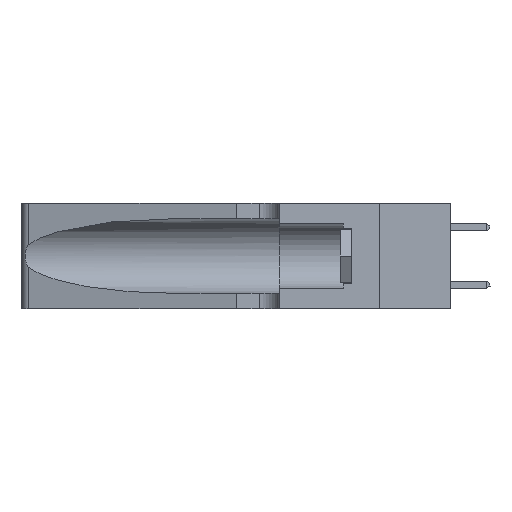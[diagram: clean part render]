
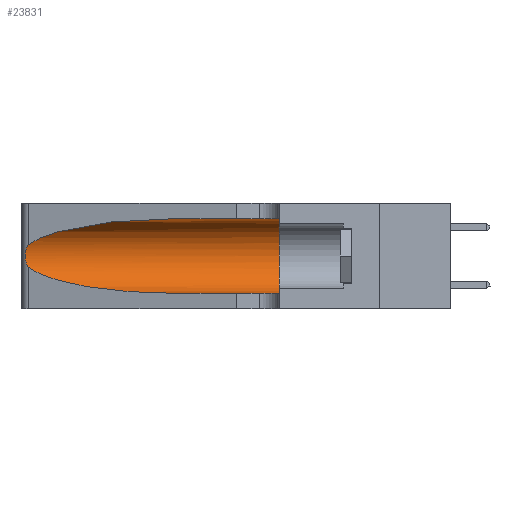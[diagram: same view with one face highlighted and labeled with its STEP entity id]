
A CAD part, left-side view. The second image highlights one B-rep face of the part: STEP entity #23831.
In plain terms, the highlighted cylindrical face has radius 3.308 mm (diameter 6.617 mm), a partial arc.
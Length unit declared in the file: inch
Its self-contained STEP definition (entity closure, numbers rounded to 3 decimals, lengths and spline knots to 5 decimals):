
#140 = ORIENTED_EDGE ( 'NONE', *, *, #17672, .T. ) ;
#595 = B_SPLINE_CURVE_WITH_KNOTS ( 'NONE', 3,
 ( #10489, #21453, #28916, #2575, #16901, #21864, #9823, #29399, #17494, #22380, #30138, #13335, #4917, #28024 ),
 .UNSPECIFIED., .F., .F.,
 ( 4, 2, 2, 2, 2, 2, 4 ),
 ( 0., 0.00027, 0.00053, 0.00107, 0.0016, 0.00187, 0.00214 ),
 .UNSPECIFIED. ) ;
#686 = AXIS2_PLACEMENT_3D ( 'NONE', #2015, #11781, #25969 ) ;
#1318 = DIRECTION ( 'NONE',  ( 0., -1., 0. ) ) ;
#2015 = CARTESIAN_POINT ( 'NONE',  ( 0.1305, 1.61858, 0.185 ) ) ;
#2575 = CARTESIAN_POINT ( 'NONE',  ( 0.25787, 1.23484, 0.2124 ) ) ;
#3003 = EDGE_CURVE ( 'NONE', #3062, #8077, #16584, .T. ) ;
#3062 = VERTEX_POINT ( 'NONE', #16203 ) ;
#3171 = ORIENTED_EDGE ( 'NONE', *, *, #3003, .F. ) ;
#3397 = VERTEX_POINT ( 'NONE', #16098 ) ;
#4917 = CARTESIAN_POINT ( 'NONE',  ( 0.25555, 1.22993, 0.14849 ) ) ;
#7480 = AXIS2_PLACEMENT_3D ( 'NONE', #28625, #30835, #21142 ) ;
#7861 = DIRECTION ( 'NONE',  ( 0., -1., 0. ) ) ;
#8012 = CARTESIAN_POINT ( 'NONE',  ( 0.2373, 1.15595, 0.28018 ) ) ;
#8077 = VERTEX_POINT ( 'NONE', #28107 ) ;
#8131 = CARTESIAN_POINT ( 'NONE',  ( 0.25487, 1.22718, 0.22369 ) ) ;
#8479 = CARTESIAN_POINT ( 'NONE',  ( 0.1305, 1.61858, 0.31525 ) ) ;
#9499 =( BOUNDED_CURVE ( )  B_SPLINE_CURVE ( 3, ( #11770, #10043, #17106, #12783 ),
 .UNSPECIFIED., .F., .T. ) 
 B_SPLINE_CURVE_WITH_KNOTS ( ( 4, 4 ),
 ( 3.44316, 4.71239 ),
 .UNSPECIFIED. ) 
 CURVE ( )  GEOMETRIC_REPRESENTATION_ITEM ( )  RATIONAL_B_SPLINE_CURVE ( ( 1., 0.87, 0.87, 1. ) ) 
 REPRESENTATION_ITEM ( '' )  );
#9823 = CARTESIAN_POINT ( 'NONE',  ( 0.26075, 1.23896, 0.19203 ) ) ;
#10043 = CARTESIAN_POINT ( 'NONE',  ( 0.2373, 1.15595, 0.08982 ) ) ;
#10489 = CARTESIAN_POINT ( 'NONE',  ( 0.25487, 1.22718, 0.22369 ) ) ;
#11770 = CARTESIAN_POINT ( 'NONE',  ( 0.25487, 1.22718, 0.14631 ) ) ;
#11781 = DIRECTION ( 'NONE',  ( 0., -1., 0. ) ) ;
#12393 = VECTOR ( 'NONE', #7861, 39.37008 ) ;
#12783 = CARTESIAN_POINT ( 'NONE',  ( 0.1305, 0.72297, 0.05475 ) ) ;
#13335 = CARTESIAN_POINT ( 'NONE',  ( 0.25639, 1.23186, 0.15144 ) ) ;
#13551 = EDGE_CURVE ( 'NONE', #17239, #24078, #9499, .T. ) ;
#13596 = ORIENTED_EDGE ( 'NONE', *, *, #28019, .T. ) ;
#14222 = EDGE_CURVE ( 'NONE', #3397, #3062, #29926, .T. ) ;
#15658 = CARTESIAN_POINT ( 'NONE',  ( 0.1305, 0.72297, 0.05475 ) ) ;
#16098 = CARTESIAN_POINT ( 'NONE',  ( 0.1305, 0.72297, 0.31525 ) ) ;
#16203 = CARTESIAN_POINT ( 'NONE',  ( 0.1305, 0.35, 0.31525 ) ) ;
#16584 = CIRCLE ( 'NONE', #7480, 0.13025 ) ;
#16759 = CYLINDRICAL_SURFACE ( 'NONE', #686, 0.13025 ) ;
#16901 = CARTESIAN_POINT ( 'NONE',  ( 0.25854, 1.2359, 0.20912 ) ) ;
#17106 = CARTESIAN_POINT ( 'NONE',  ( 0.18966, 0.96281, 0.05475 ) ) ;
#17239 = VERTEX_POINT ( 'NONE', #25004 ) ;
#17494 = CARTESIAN_POINT ( 'NONE',  ( 0.26017, 1.23833, 0.17102 ) ) ;
#17672 = EDGE_CURVE ( 'NONE', #20679, #17239, #595, .T. ) ;
#18818 = LINE ( 'NONE', #22119, #12393 ) ;
#20454 = CARTESIAN_POINT ( 'NONE',  ( 0.1305, 0.72297, 0.31525 ) ) ;
#20679 = VERTEX_POINT ( 'NONE', #21234 ) ;
#20859 = EDGE_LOOP ( 'NONE', ( #23360, #140, #28391, #13596, #3171, #23961 ) ) ;
#21142 = DIRECTION ( 'NONE',  ( 0., 0., 1. ) ) ;
#21234 = CARTESIAN_POINT ( 'NONE',  ( 0.25487, 1.22718, 0.22369 ) ) ;
#21453 = CARTESIAN_POINT ( 'NONE',  ( 0.25555, 1.22994, 0.2215 ) ) ;
#21864 = CARTESIAN_POINT ( 'NONE',  ( 0.26018, 1.23835, 0.19895 ) ) ;
#22119 = CARTESIAN_POINT ( 'NONE',  ( 0.1305, 1.61858, 0.05475 ) ) ;
#22380 = CARTESIAN_POINT ( 'NONE',  ( 0.25856, 1.23593, 0.16098 ) ) ;
#22589 = CARTESIAN_POINT ( 'NONE',  ( 0.18966, 0.96281, 0.31525 ) ) ;
#23360 = ORIENTED_EDGE ( 'NONE', *, *, #23929, .T. ) ;
#23831 = ADVANCED_FACE ( 'NONE', ( #29248 ), #16759, .F. ) ;
#23929 = EDGE_CURVE ( 'NONE', #3397, #20679, #25993, .T. ) ;
#23961 = ORIENTED_EDGE ( 'NONE', *, *, #14222, .F. ) ;
#24078 = VERTEX_POINT ( 'NONE', #15658 ) ;
#25004 = CARTESIAN_POINT ( 'NONE',  ( 0.25487, 1.22718, 0.14631 ) ) ;
#25969 = DIRECTION ( 'NONE',  ( 0., 0., -1. ) ) ;
#25993 =( BOUNDED_CURVE ( )  B_SPLINE_CURVE ( 3, ( #20454, #22589, #8012, #8131 ),
 .UNSPECIFIED., .F., .F. ) 
 B_SPLINE_CURVE_WITH_KNOTS ( ( 4, 4 ),
 ( 1.5708, 2.84003 ),
 .UNSPECIFIED. ) 
 CURVE ( )  GEOMETRIC_REPRESENTATION_ITEM ( )  RATIONAL_B_SPLINE_CURVE ( ( 1., 0.87, 0.87, 1. ) ) 
 REPRESENTATION_ITEM ( '' )  );
#26533 = VECTOR ( 'NONE', #1318, 39.37008 ) ;
#28019 = EDGE_CURVE ( 'NONE', #24078, #8077, #18818, .T. ) ;
#28024 = CARTESIAN_POINT ( 'NONE',  ( 0.25487, 1.22718, 0.14631 ) ) ;
#28107 = CARTESIAN_POINT ( 'NONE',  ( 0.1305, 0.35, 0.05475 ) ) ;
#28391 = ORIENTED_EDGE ( 'NONE', *, *, #13551, .T. ) ;
#28625 = CARTESIAN_POINT ( 'NONE',  ( 0.1305, 0.35, 0.185 ) ) ;
#28916 = CARTESIAN_POINT ( 'NONE',  ( 0.25639, 1.23184, 0.21858 ) ) ;
#29248 = FACE_OUTER_BOUND ( 'NONE', #20859, .T. ) ;
#29399 = CARTESIAN_POINT ( 'NONE',  ( 0.26075, 1.23896, 0.178 ) ) ;
#29926 = LINE ( 'NONE', #8479, #26533 ) ;
#30138 = CARTESIAN_POINT ( 'NONE',  ( 0.25789, 1.23486, 0.15765 ) ) ;
#30835 = DIRECTION ( 'NONE',  ( 0., 1., 0. ) ) ;
